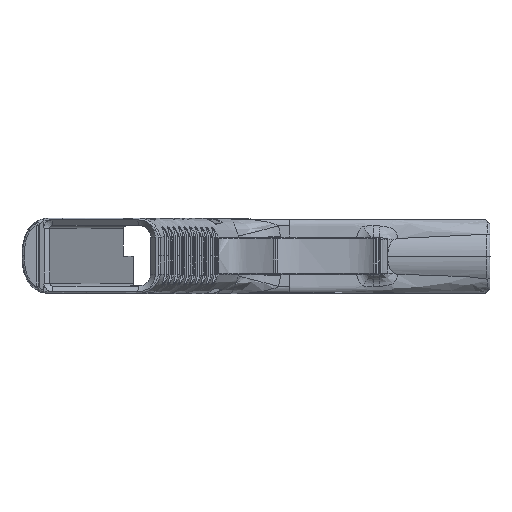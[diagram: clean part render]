
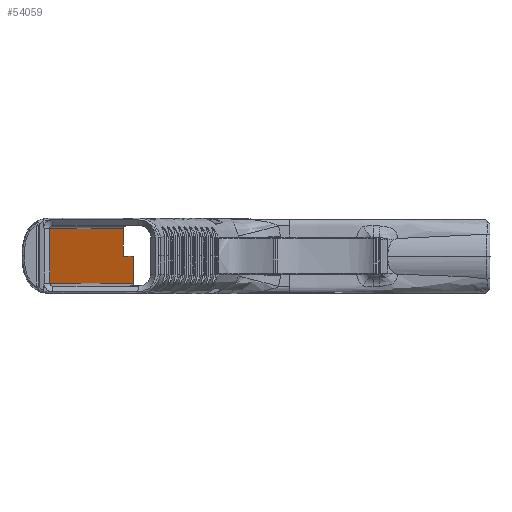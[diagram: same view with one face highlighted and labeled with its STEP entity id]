
A CAD part, top view. The second image highlights one B-rep face of the part: STEP entity #54059.
In plain terms, the highlighted planar face has unit normal (0.951, 0, 0.309).
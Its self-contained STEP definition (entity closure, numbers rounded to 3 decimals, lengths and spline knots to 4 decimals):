
#1638 = VECTOR ( 'NONE', #37184, 39.3701 ) ;
#1756 = VERTEX_POINT ( 'NONE', #112474 ) ;
#2473 = CARTESIAN_POINT ( 'NONE',  ( 1.9466, 0.0001, -3.4826 ) ) ;
#3792 = LINE ( 'NONE', #7697, #101774 ) ;
#7697 = CARTESIAN_POINT ( 'NONE',  ( 2.0746, 0.37, -3.8765 ) ) ;
#9336 = DIRECTION ( 'NONE',  ( 0.309, 0., -0.951 ) ) ;
#9358 = ORIENTED_EDGE ( 'NONE', *, *, #17774, .F. ) ;
#9559 = EDGE_CURVE ( 'NONE', #113464, #47801, #32819, .T. ) ;
#10566 = VECTOR ( 'NONE', #90387, 39.3701 ) ;
#15358 = DIRECTION ( 'NONE',  ( -0.309, 0., 0.951 ) ) ;
#15584 = LINE ( 'NONE', #76621, #67400 ) ;
#17774 = EDGE_CURVE ( 'NONE', #90404, #61174, #3792, .T. ) ;
#23936 = LINE ( 'NONE', #100670, #80256 ) ;
#24010 = ORIENTED_EDGE ( 'NONE', *, *, #45043, .F. ) ;
#32819 = LINE ( 'NONE', #44700, #10566 ) ;
#34812 = EDGE_LOOP ( 'NONE', ( #24010, #9358, #53109, #41222, #71861, #49999 ) ) ;
#35269 = EDGE_CURVE ( 'NONE', #96028, #113464, #15584, .T. ) ;
#37184 = DIRECTION ( 'NONE',  ( 0., -1., 0. ) ) ;
#40566 = LINE ( 'NONE', #78149, #79167 ) ;
#41222 = ORIENTED_EDGE ( 'NONE', *, *, #78228, .F. ) ;
#44700 = CARTESIAN_POINT ( 'NONE',  ( 2.0809, 0., -3.896 ) ) ;
#45043 = EDGE_CURVE ( 'NONE', #61174, #96028, #92263, .T. ) ;
#46753 = CARTESIAN_POINT ( 'NONE',  ( 1.9466, 0., -3.4826 ) ) ;
#47196 = DIRECTION ( 'NONE',  ( 0.309, 0., -0.951 ) ) ;
#47801 = VERTEX_POINT ( 'NONE', #118361 ) ;
#49999 = ORIENTED_EDGE ( 'NONE', *, *, #35269, .F. ) ;
#52666 = CARTESIAN_POINT ( 'NONE',  ( 2.0809, 0.0001, -3.896 ) ) ;
#53109 = ORIENTED_EDGE ( 'NONE', *, *, #57779, .F. ) ;
#54059 = ADVANCED_FACE ( 'NONE', ( #70552 ), #72160, .F. ) ;
#57779 = EDGE_CURVE ( 'NONE', #1756, #90404, #40566, .T. ) ;
#61174 = VERTEX_POINT ( 'NONE', #82143 ) ;
#67400 = VECTOR ( 'NONE', #47196, 39.3701 ) ;
#69579 = CARTESIAN_POINT ( 'NONE',  ( 0.9499, 0.37, -0.4151 ) ) ;
#70552 = FACE_OUTER_BOUND ( 'NONE', #34812, .T. ) ;
#71861 = ORIENTED_EDGE ( 'NONE', *, *, #9559, .F. ) ;
#72160 = PLANE ( 'NONE',  #114362 ) ;
#76621 = CARTESIAN_POINT ( 'NONE',  ( 2.0746, 0.0001, -3.8765 ) ) ;
#78149 = CARTESIAN_POINT ( 'NONE',  ( 0.9499, 0., -0.4151 ) ) ;
#78228 = EDGE_CURVE ( 'NONE', #47801, #1756, #23936, .T. ) ;
#79167 = VECTOR ( 'NONE', #85616, 39.3701 ) ;
#80256 = VECTOR ( 'NONE', #122162, 39.3701 ) ;
#81324 = CARTESIAN_POINT ( 'NONE',  ( 2.0746, 0., -3.8765 ) ) ;
#82143 = CARTESIAN_POINT ( 'NONE',  ( 1.9466, 0.37, -3.4826 ) ) ;
#85616 = DIRECTION ( 'NONE',  ( 0., 1., 0. ) ) ;
#90387 = DIRECTION ( 'NONE',  ( 0., -1., 0. ) ) ;
#90404 = VERTEX_POINT ( 'NONE', #69579 ) ;
#92263 = LINE ( 'NONE', #46753, #1638 ) ;
#96028 = VERTEX_POINT ( 'NONE', #2473 ) ;
#100670 = CARTESIAN_POINT ( 'NONE',  ( 2.0746, -0.37, -3.8765 ) ) ;
#101774 = VECTOR ( 'NONE', #9336, 39.3701 ) ;
#112474 = CARTESIAN_POINT ( 'NONE',  ( 0.9499, -0.37, -0.4151 ) ) ;
#113464 = VERTEX_POINT ( 'NONE', #52666 ) ;
#114362 = AXIS2_PLACEMENT_3D ( 'NONE', #81324, #119500, #15358 ) ;
#118361 = CARTESIAN_POINT ( 'NONE',  ( 2.0809, -0.37, -3.896 ) ) ;
#119500 = DIRECTION ( 'NONE',  ( -0.951, 0., -0.309 ) ) ;
#122162 = DIRECTION ( 'NONE',  ( -0.309, 0., 0.951 ) ) ;
